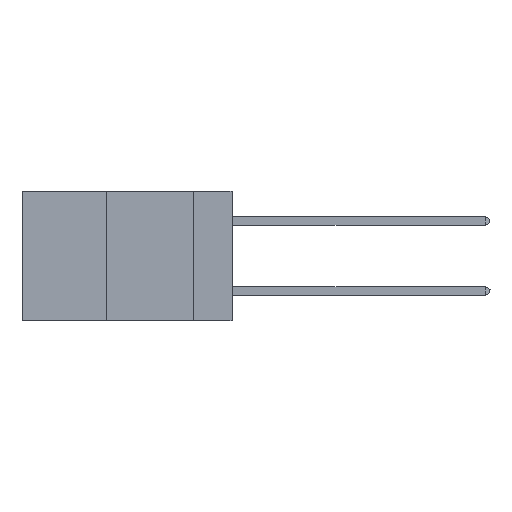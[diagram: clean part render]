
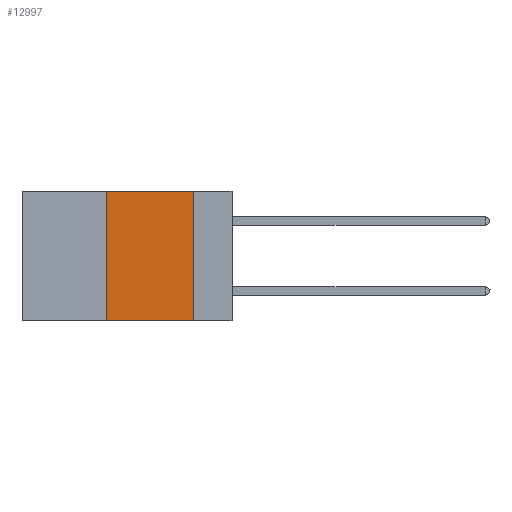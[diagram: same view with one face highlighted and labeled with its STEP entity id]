
A CAD part, left-side view. The second image highlights one B-rep face of the part: STEP entity #12997.
In plain terms, the highlighted planar face has unit normal (-1, 0, 0).
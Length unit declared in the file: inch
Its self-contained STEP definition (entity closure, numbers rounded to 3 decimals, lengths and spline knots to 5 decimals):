
#1579 = VERTEX_POINT ( 'NONE', #4241 ) ;
#2543 = EDGE_CURVE ( 'NONE', #1579, #14755, #23148, .T. ) ;
#3931 = CARTESIAN_POINT ( 'NONE',  ( 0., 0.36, 0. ) ) ;
#4241 = CARTESIAN_POINT ( 'NONE',  ( 0., 0.36, -0.37 ) ) ;
#5428 = EDGE_LOOP ( 'NONE', ( #29588, #18588, #20362, #26390 ) ) ;
#5796 = VECTOR ( 'NONE', #15674, 39.37008 ) ;
#5823 = EDGE_CURVE ( 'NONE', #1579, #13646, #26703, .T. ) ;
#6172 = DIRECTION ( 'NONE',  ( 0., 0., -1. ) ) ;
#9655 = CARTESIAN_POINT ( 'NONE',  ( 0., 0.11, 0. ) ) ;
#11523 = PLANE ( 'NONE',  #18008 ) ;
#12524 = FACE_OUTER_BOUND ( 'NONE', #5428, .T. ) ;
#12997 = ADVANCED_FACE ( 'NONE', ( #12524 ), #11523, .F. ) ;
#13145 = DIRECTION ( 'NONE',  ( 0., -1., 0. ) ) ;
#13247 = CARTESIAN_POINT ( 'NONE',  ( 0., 0.6, -0.37 ) ) ;
#13646 = VERTEX_POINT ( 'NONE', #19298 ) ;
#14033 = DIRECTION ( 'NONE',  ( 1., 0., 0. ) ) ;
#14755 = VERTEX_POINT ( 'NONE', #27029 ) ;
#15674 = DIRECTION ( 'NONE',  ( 0., 0., 1. ) ) ;
#15989 = LINE ( 'NONE', #23018, #20107 ) ;
#16014 = DIRECTION ( 'NONE',  ( 0., -1., 0. ) ) ;
#16343 = CARTESIAN_POINT ( 'NONE',  ( 0., 0.6, 0. ) ) ;
#17182 = VECTOR ( 'NONE', #13145, 39.37008 ) ;
#18008 = AXIS2_PLACEMENT_3D ( 'NONE', #16343, #14033, #28251 ) ;
#18588 = ORIENTED_EDGE ( 'NONE', *, *, #28996, .F. ) ;
#19298 = CARTESIAN_POINT ( 'NONE',  ( 0., 0.36, 0. ) ) ;
#20107 = VECTOR ( 'NONE', #16014, 39.37008 ) ;
#20268 = CARTESIAN_POINT ( 'NONE',  ( 0., 0.11, 0. ) ) ;
#20362 = ORIENTED_EDGE ( 'NONE', *, *, #5823, .F. ) ;
#23018 = CARTESIAN_POINT ( 'NONE',  ( 0., 0.6, 0. ) ) ;
#23070 = VERTEX_POINT ( 'NONE', #9655 ) ;
#23148 = LINE ( 'NONE', #13247, #17182 ) ;
#25371 = VECTOR ( 'NONE', #6172, 39.37008 ) ;
#26390 = ORIENTED_EDGE ( 'NONE', *, *, #2543, .T. ) ;
#26472 = LINE ( 'NONE', #20268, #25371 ) ;
#26703 = LINE ( 'NONE', #3931, #5796 ) ;
#27029 = CARTESIAN_POINT ( 'NONE',  ( 0., 0.11, -0.37 ) ) ;
#28251 = DIRECTION ( 'NONE',  ( 0., 0., -1. ) ) ;
#28996 = EDGE_CURVE ( 'NONE', #13646, #23070, #15989, .T. ) ;
#29588 = ORIENTED_EDGE ( 'NONE', *, *, #29885, .F. ) ;
#29885 = EDGE_CURVE ( 'NONE', #23070, #14755, #26472, .T. ) ;
